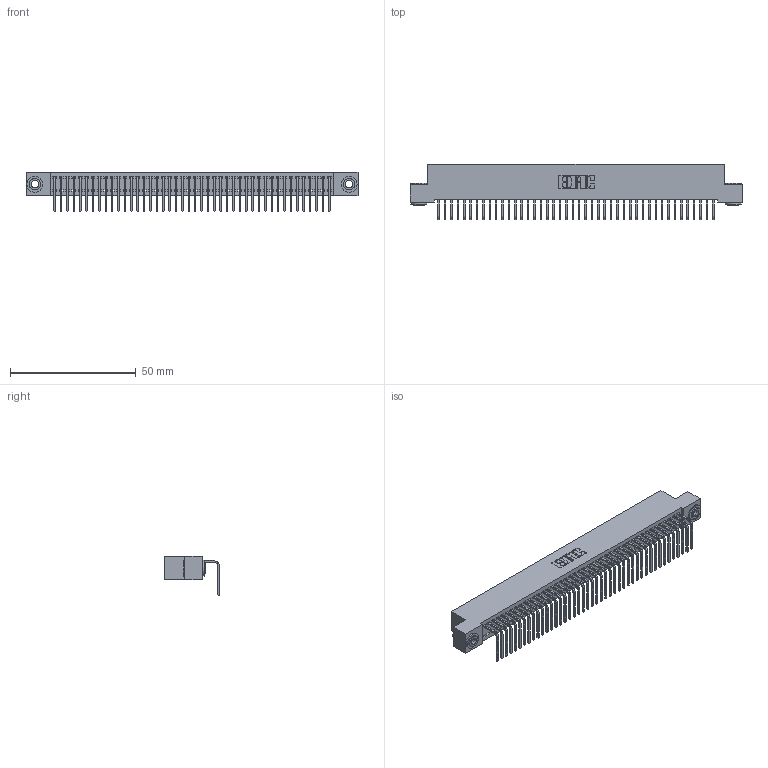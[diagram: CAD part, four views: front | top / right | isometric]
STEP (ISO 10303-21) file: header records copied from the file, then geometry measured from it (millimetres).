
FILE_DESCRIPTION (( 'STEP AP203' ), '1' );
FILE_NAME ('392-044-558-103.STEP', '2019-10-07T22:39:46', ( '' ), ( '' ), 'SwSTEP 2.0', 'SolidWorks 2016', '' );
FILE_SCHEMA (( 'CONFIG_CONTROL_DESIGN' ));
Length unit declared in the file: inch
Products named in the file (4): 345-292-001_558 Tail - 2; 342-250-002_345-250-002-102; 392-044-558-103; 342 Part_.156 TH
Assembly tree (47 placements, depth 2):
  392-044-558-103
    342 Part_.156 TH
    345-292-001_558 Tail - 2  x44
    342-250-002_345-250-002-102  x2
Bounding box: 132.08 x 21.91 x 15.62 mm (x, y, z)
Volume: 11757.6 mm3; surface area: 18361.5 mm2
Topology: 47 solids, 47 shells, 2788 faces, 8383 edges, 5526 vertices
Faces by surface type: plane 2012, cylinder 768, cone 8
Entity records: 27242 total; most frequent: CARTESIAN_POINT 4677, ORIENTED_EDGE 4650, DIRECTION 3975, EDGE_CURVE 2325, VECTOR 2173, LINE 2173, VERTEX_POINT 1546, AXIS2_PLACEMENT_3D 901
